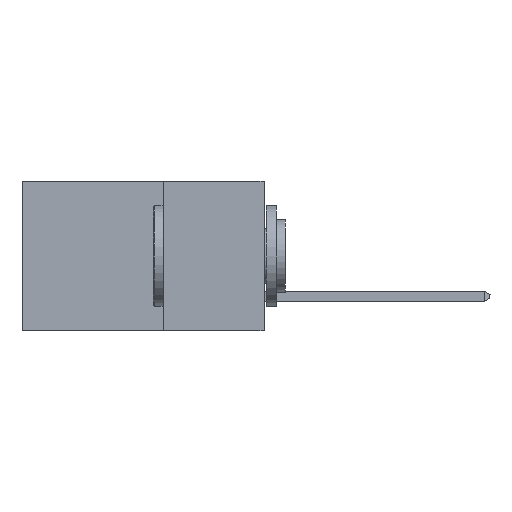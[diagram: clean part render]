
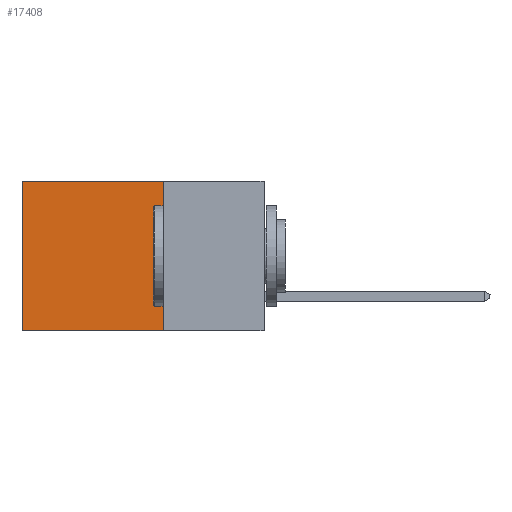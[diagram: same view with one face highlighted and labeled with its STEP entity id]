
A CAD part, left-side view. The second image highlights one B-rep face of the part: STEP entity #17408.
In plain terms, the highlighted planar face has unit normal (-1, 0, 0).
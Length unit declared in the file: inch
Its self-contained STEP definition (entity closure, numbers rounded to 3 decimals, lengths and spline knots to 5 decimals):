
#1661 = LINE ( 'NONE', #13940, #5658 ) ;
#2376 = VERTEX_POINT ( 'NONE', #19589 ) ;
#2603 = VERTEX_POINT ( 'NONE', #3639 ) ;
#3346 = LINE ( 'NONE', #10309, #5233 ) ;
#3447 = ORIENTED_EDGE ( 'NONE', *, *, #12316, .T. ) ;
#3639 = CARTESIAN_POINT ( 'NONE',  ( 0.2615, 0.6, 0. ) ) ;
#4662 = DIRECTION ( 'NONE',  ( 0., 0., -1. ) ) ;
#5009 = CARTESIAN_POINT ( 'NONE',  ( 0.2615, 0.25, -0.37 ) ) ;
#5233 = VECTOR ( 'NONE', #12452, 39.37008 ) ;
#5658 = VECTOR ( 'NONE', #20895, 39.37008 ) ;
#6374 = PLANE ( 'NONE',  #19916 ) ;
#7306 = ORIENTED_EDGE ( 'NONE', *, *, #11068, .T. ) ;
#7341 = CARTESIAN_POINT ( 'NONE',  ( 0.2615, 0.6, -0.37 ) ) ;
#8083 = DIRECTION ( 'NONE',  ( 1., 0., 0. ) ) ;
#9489 = CARTESIAN_POINT ( 'NONE',  ( 0.2615, 0.25, -0.37 ) ) ;
#9914 = LINE ( 'NONE', #9489, #11092 ) ;
#10297 = EDGE_CURVE ( 'NONE', #14578, #2376, #3346, .T. ) ;
#10309 = CARTESIAN_POINT ( 'NONE',  ( 0.2615, 0.25, -0.37 ) ) ;
#10380 = VERTEX_POINT ( 'NONE', #7341 ) ;
#11056 = DIRECTION ( 'NONE',  ( 0., 0., -1. ) ) ;
#11068 = EDGE_CURVE ( 'NONE', #2603, #10380, #12747, .T. ) ;
#11092 = VECTOR ( 'NONE', #11722, 39.37008 ) ;
#11618 = EDGE_CURVE ( 'NONE', #2376, #10380, #9914, .T. ) ;
#11722 = DIRECTION ( 'NONE',  ( 0., 1., 0. ) ) ;
#12316 = EDGE_CURVE ( 'NONE', #14578, #2603, #1661, .T. ) ;
#12452 = DIRECTION ( 'NONE',  ( 0., 0., -1. ) ) ;
#12747 = LINE ( 'NONE', #19694, #21232 ) ;
#13940 = CARTESIAN_POINT ( 'NONE',  ( 0.2615, 0.25, 0. ) ) ;
#14578 = VERTEX_POINT ( 'NONE', #17656 ) ;
#14938 = EDGE_LOOP ( 'NONE', ( #7306, #19451, #18122, #3447 ) ) ;
#17408 = ADVANCED_FACE ( 'NONE', ( #21960 ), #6374, .F. ) ;
#17656 = CARTESIAN_POINT ( 'NONE',  ( 0.2615, 0.25, 0. ) ) ;
#18122 = ORIENTED_EDGE ( 'NONE', *, *, #10297, .F. ) ;
#19451 = ORIENTED_EDGE ( 'NONE', *, *, #11618, .F. ) ;
#19589 = CARTESIAN_POINT ( 'NONE',  ( 0.2615, 0.25, -0.37 ) ) ;
#19694 = CARTESIAN_POINT ( 'NONE',  ( 0.2615, 0.6, -0.37 ) ) ;
#19916 = AXIS2_PLACEMENT_3D ( 'NONE', #5009, #8083, #4662 ) ;
#20895 = DIRECTION ( 'NONE',  ( 0., 1., 0. ) ) ;
#21232 = VECTOR ( 'NONE', #11056, 39.37008 ) ;
#21960 = FACE_OUTER_BOUND ( 'NONE', #14938, .T. ) ;
